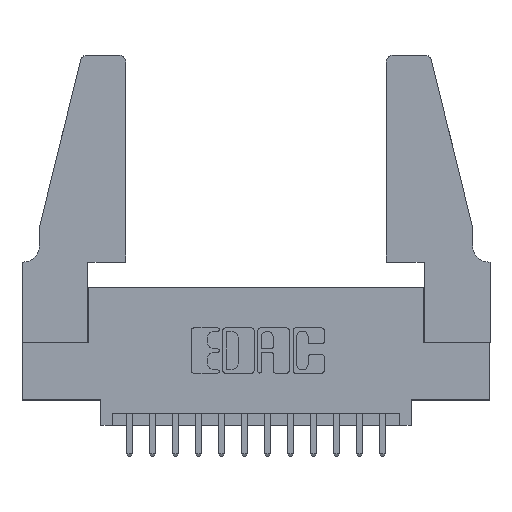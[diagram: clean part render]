
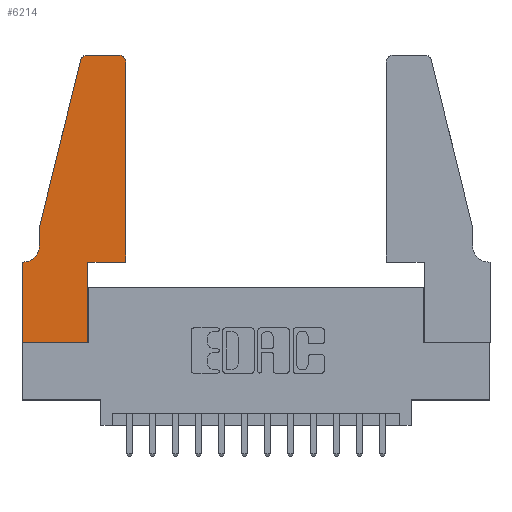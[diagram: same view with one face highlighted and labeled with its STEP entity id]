
A CAD part, top view. The second image highlights one B-rep face of the part: STEP entity #6214.
In plain terms, the highlighted planar face has unit normal (0, 0, 1).
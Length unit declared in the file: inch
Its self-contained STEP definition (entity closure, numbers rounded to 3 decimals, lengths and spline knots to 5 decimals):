
#175 = EDGE_CURVE ( 'NONE', #12277, #5617, #13332, .T. ) ;
#225 = EDGE_CURVE ( 'NONE', #10227, #1230, #9709, .T. ) ;
#248 = CIRCLE ( 'NONE', #11803, 0.07 ) ;
#305 = CARTESIAN_POINT ( 'NONE',  ( 0.284, 1.22, 0.37 ) ) ;
#486 = ORIENTED_EDGE ( 'NONE', *, *, #175, .T. ) ;
#831 = CARTESIAN_POINT ( 'NONE',  ( 0.4505, 1.22, 0.37 ) ) ;
#862 = EDGE_LOOP ( 'NONE', ( #8814, #12812, #8396, #13527, #4158, #7265, #13454, #4725, #9319, #6487, #10805, #486 ) ) ;
#1108 = EDGE_CURVE ( 'NONE', #15707, #10227, #1132, .T. ) ;
#1132 = LINE ( 'NONE', #6370, #7984 ) ;
#1230 = VERTEX_POINT ( 'NONE', #11427 ) ;
#1260 = EDGE_CURVE ( 'NONE', #6941, #14707, #13863, .T. ) ;
#1320 = CARTESIAN_POINT ( 'NONE',  ( 0.284, 1.25, 0.37 ) ) ;
#1614 = CARTESIAN_POINT ( 'NONE',  ( 0.0755, 0.35, 0.37 ) ) ;
#1635 = CARTESIAN_POINT ( 'NONE',  ( 0.0755, 0.5, 0.37 ) ) ;
#2062 = CARTESIAN_POINT ( 'NONE',  ( 0., 0., 0.37 ) ) ;
#2203 = AXIS2_PLACEMENT_3D ( 'NONE', #305, #10020, #6465 ) ;
#2463 = VECTOR ( 'NONE', #8409, 39.37008 ) ;
#2526 = AXIS2_PLACEMENT_3D ( 'NONE', #13722, #7675, #12443 ) ;
#2559 = CARTESIAN_POINT ( 'NONE',  ( 0., 0., 0.37 ) ) ;
#2591 = VERTEX_POINT ( 'NONE', #10293 ) ;
#2595 = CARTESIAN_POINT ( 'NONE',  ( 0.0755, 0.42, 0.37 ) ) ;
#2857 = DIRECTION ( 'NONE',  ( -1., 0., 0. ) ) ;
#3012 = VECTOR ( 'NONE', #4128, 39.37008 ) ;
#3126 = EDGE_CURVE ( 'NONE', #13025, #11465, #6375, .T. ) ;
#3200 = DIRECTION ( 'NONE',  ( 0., 0., -1. ) ) ;
#3376 = AXIS2_PLACEMENT_3D ( 'NONE', #14105, #9377, #14325 ) ;
#3953 = PLANE ( 'NONE',  #2526 ) ;
#4128 = DIRECTION ( 'NONE',  ( 0., -1., 0. ) ) ;
#4158 = ORIENTED_EDGE ( 'NONE', *, *, #15619, .T. ) ;
#4725 = ORIENTED_EDGE ( 'NONE', *, *, #8113, .T. ) ;
#4740 = VECTOR ( 'NONE', #7899, 39.37008 ) ;
#5116 = VECTOR ( 'NONE', #6667, 39.37008 ) ;
#5202 = VERTEX_POINT ( 'NONE', #1320 ) ;
#5617 = VERTEX_POINT ( 'NONE', #12173 ) ;
#5787 = CARTESIAN_POINT ( 'NONE',  ( 0.0055, 0.35, 0.37 ) ) ;
#5906 = LINE ( 'NONE', #6882, #4740 ) ;
#6058 = VECTOR ( 'NONE', #6637, 39.37008 ) ;
#6214 = ADVANCED_FACE ( 'NONE', ( #7908 ), #3953, .T. ) ;
#6288 = VECTOR ( 'NONE', #9624, 39.37008 ) ;
#6370 = CARTESIAN_POINT ( 'NONE',  ( 0.2865, 0.35, 0.37 ) ) ;
#6375 = LINE ( 'NONE', #2062, #13253 ) ;
#6465 = DIRECTION ( 'NONE',  ( 1., 0., 0. ) ) ;
#6487 = ORIENTED_EDGE ( 'NONE', *, *, #225, .T. ) ;
#6637 = DIRECTION ( 'NONE',  ( 1., 0., 0. ) ) ;
#6667 = DIRECTION ( 'NONE',  ( 0., 1., 0. ) ) ;
#6882 = CARTESIAN_POINT ( 'NONE',  ( 0.2605, 1.25, 0.37 ) ) ;
#6941 = VERTEX_POINT ( 'NONE', #15259 ) ;
#6960 = EDGE_CURVE ( 'NONE', #1230, #12277, #9878, .T. ) ;
#6979 = LINE ( 'NONE', #1614, #11758 ) ;
#6989 = EDGE_CURVE ( 'NONE', #5617, #5202, #5906, .T. ) ;
#7265 = ORIENTED_EDGE ( 'NONE', *, *, #8918, .T. ) ;
#7551 = DIRECTION ( 'NONE',  ( 0., 1., 0. ) ) ;
#7564 = LINE ( 'NONE', #13912, #6058 ) ;
#7675 = DIRECTION ( 'NONE',  ( 0., 0., 1. ) ) ;
#7899 = DIRECTION ( 'NONE',  ( -1., 0., 0. ) ) ;
#7908 = FACE_OUTER_BOUND ( 'NONE', #862, .T. ) ;
#7984 = VECTOR ( 'NONE', #7551, 39.37008 ) ;
#8113 = EDGE_CURVE ( 'NONE', #11465, #15707, #7564, .T. ) ;
#8396 = ORIENTED_EDGE ( 'NONE', *, *, #8430, .T. ) ;
#8409 = DIRECTION ( 'NONE',  ( -0.239, -0.971, 0. ) ) ;
#8430 = EDGE_CURVE ( 'NONE', #2591, #6941, #8912, .T. ) ;
#8777 = VERTEX_POINT ( 'NONE', #5787 ) ;
#8814 = ORIENTED_EDGE ( 'NONE', *, *, #6989, .T. ) ;
#8912 = LINE ( 'NONE', #1635, #2463 ) ;
#8918 = EDGE_CURVE ( 'NONE', #8777, #13025, #6979, .T. ) ;
#9319 = ORIENTED_EDGE ( 'NONE', *, *, #1108, .T. ) ;
#9377 = DIRECTION ( 'NONE',  ( 0., 0., 1. ) ) ;
#9579 = CARTESIAN_POINT ( 'NONE',  ( 0.4505, 0.35, 0.37 ) ) ;
#9624 = DIRECTION ( 'NONE',  ( 1., 0., 0. ) ) ;
#9709 = LINE ( 'NONE', #9579, #6288 ) ;
#9878 = LINE ( 'NONE', #13947, #5116 ) ;
#10020 = DIRECTION ( 'NONE',  ( 0., 0., 1. ) ) ;
#10227 = VERTEX_POINT ( 'NONE', #14936 ) ;
#10293 = CARTESIAN_POINT ( 'NONE',  ( 0.25487, 1.22718, 0.37 ) ) ;
#10805 = ORIENTED_EDGE ( 'NONE', *, *, #6960, .T. ) ;
#11427 = CARTESIAN_POINT ( 'NONE',  ( 0.4505, 0.35, 0.37 ) ) ;
#11465 = VERTEX_POINT ( 'NONE', #2559 ) ;
#11607 = CARTESIAN_POINT ( 'NONE',  ( 0.0055, 0.42, 0.37 ) ) ;
#11758 = VECTOR ( 'NONE', #2857, 39.37008 ) ;
#11803 = AXIS2_PLACEMENT_3D ( 'NONE', #11607, #3200, #12708 ) ;
#12173 = CARTESIAN_POINT ( 'NONE',  ( 0.4205, 1.25, 0.37 ) ) ;
#12277 = VERTEX_POINT ( 'NONE', #831 ) ;
#12373 = CARTESIAN_POINT ( 'NONE',  ( 0., 0.35, 0.37 ) ) ;
#12443 = DIRECTION ( 'NONE',  ( 1., 0., 0. ) ) ;
#12708 = DIRECTION ( 'NONE',  ( -1., 0., 0. ) ) ;
#12812 = ORIENTED_EDGE ( 'NONE', *, *, #13201, .T. ) ;
#12966 = DIRECTION ( 'NONE',  ( 0., -1., 0. ) ) ;
#13025 = VERTEX_POINT ( 'NONE', #12373 ) ;
#13201 = EDGE_CURVE ( 'NONE', #5202, #2591, #15377, .T. ) ;
#13253 = VECTOR ( 'NONE', #12966, 39.37008 ) ;
#13332 = CIRCLE ( 'NONE', #3376, 0.03 ) ;
#13454 = ORIENTED_EDGE ( 'NONE', *, *, #3126, .T. ) ;
#13527 = ORIENTED_EDGE ( 'NONE', *, *, #1260, .T. ) ;
#13722 = CARTESIAN_POINT ( 'NONE',  ( 0., 0.35, 0.37 ) ) ;
#13831 = CARTESIAN_POINT ( 'NONE',  ( 0.2865, 0., 0.37 ) ) ;
#13863 = LINE ( 'NONE', #15059, #3012 ) ;
#13912 = CARTESIAN_POINT ( 'NONE',  ( 0., 0., 0.37 ) ) ;
#13947 = CARTESIAN_POINT ( 'NONE',  ( 0.4505, 0.35, 0.37 ) ) ;
#14105 = CARTESIAN_POINT ( 'NONE',  ( 0.4205, 1.22, 0.37 ) ) ;
#14325 = DIRECTION ( 'NONE',  ( 1., 0., 0. ) ) ;
#14707 = VERTEX_POINT ( 'NONE', #2595 ) ;
#14936 = CARTESIAN_POINT ( 'NONE',  ( 0.2865, 0.35, 0.37 ) ) ;
#15059 = CARTESIAN_POINT ( 'NONE',  ( 0.0755, 0.5, 0.37 ) ) ;
#15259 = CARTESIAN_POINT ( 'NONE',  ( 0.0755, 0.5, 0.37 ) ) ;
#15377 = CIRCLE ( 'NONE', #2203, 0.03 ) ;
#15619 = EDGE_CURVE ( 'NONE', #14707, #8777, #248, .T. ) ;
#15707 = VERTEX_POINT ( 'NONE', #13831 ) ;
